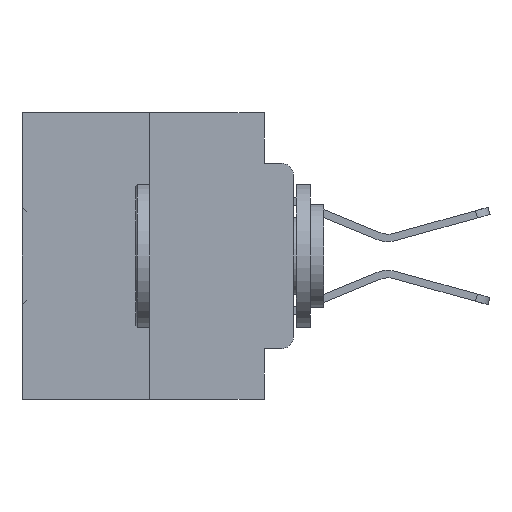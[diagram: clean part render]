
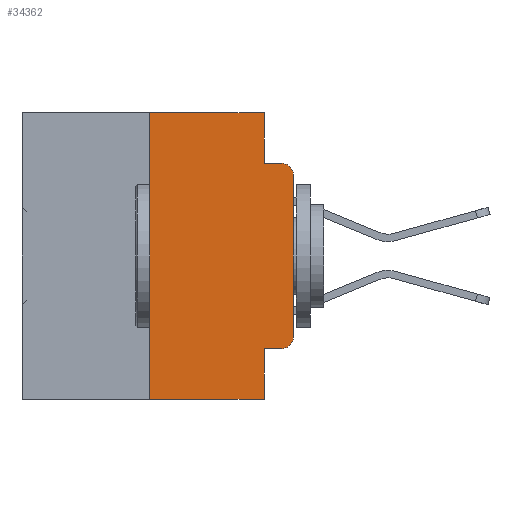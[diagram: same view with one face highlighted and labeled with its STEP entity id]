
A CAD part, left-side view. The second image highlights one B-rep face of the part: STEP entity #34362.
In plain terms, the highlighted planar face has unit normal (-1, 0, 0).
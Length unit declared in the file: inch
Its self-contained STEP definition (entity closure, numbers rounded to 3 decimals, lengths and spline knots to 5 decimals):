
#99 = DIRECTION ( 'NONE',  ( 0., 0., 1. ) ) ;
#336 = VECTOR ( 'NONE', #27512, 39.37008 ) ;
#488 = ORIENTED_EDGE ( 'NONE', *, *, #18316, .F. ) ;
#864 = CARTESIAN_POINT ( 'NONE',  ( 0., 0.25, 0. ) ) ;
#1005 = CIRCLE ( 'NONE', #3862, 0.02 ) ;
#1542 = CARTESIAN_POINT ( 'NONE',  ( 0., 0.051, -0.4115 ) ) ;
#1606 = LINE ( 'NONE', #27075, #15407 ) ;
#1761 = CARTESIAN_POINT ( 'NONE',  ( 0., 0.473, 0. ) ) ;
#2473 = CARTESIAN_POINT ( 'NONE',  ( 0., 0.051, -0.0885 ) ) ;
#3862 = AXIS2_PLACEMENT_3D ( 'NONE', #26338, #10183, #29022 ) ;
#4087 = CARTESIAN_POINT ( 'NONE',  ( 0., 0.051, -0.5 ) ) ;
#4309 = LINE ( 'NONE', #27183, #23450 ) ;
#4738 = EDGE_CURVE ( 'NONE', #10977, #25583, #14763, .T. ) ;
#4956 = VERTEX_POINT ( 'NONE', #8646 ) ;
#5624 = DIRECTION ( 'NONE',  ( 0., -1., 0. ) ) ;
#5842 = CARTESIAN_POINT ( 'NONE',  ( 0., 0.25, 0. ) ) ;
#5891 = CARTESIAN_POINT ( 'NONE',  ( 0., 0., -0.1085 ) ) ;
#7770 = EDGE_CURVE ( 'NONE', #33714, #25583, #26780, .T. ) ;
#7923 = FACE_OUTER_BOUND ( 'NONE', #13157, .T. ) ;
#8646 = CARTESIAN_POINT ( 'NONE',  ( 0., 0.051, 0. ) ) ;
#9098 = PLANE ( 'NONE',  #11448 ) ;
#9118 = EDGE_CURVE ( 'NONE', #9549, #9960, #34623, .T. ) ;
#9549 = VERTEX_POINT ( 'NONE', #18414 ) ;
#9716 = DIRECTION ( 'NONE',  ( 0., 0., -1. ) ) ;
#9960 = VERTEX_POINT ( 'NONE', #864 ) ;
#10183 = DIRECTION ( 'NONE',  ( -1., 0., 0. ) ) ;
#10211 = DIRECTION ( 'NONE',  ( -1., 0., 0. ) ) ;
#10331 = LINE ( 'NONE', #15131, #23854 ) ;
#10973 = VECTOR ( 'NONE', #23343, 39.37008 ) ;
#10977 = VERTEX_POINT ( 'NONE', #2473 ) ;
#11111 = VERTEX_POINT ( 'NONE', #30180 ) ;
#11183 = CARTESIAN_POINT ( 'NONE',  ( 0., 0.473, -0.5 ) ) ;
#11448 = AXIS2_PLACEMENT_3D ( 'NONE', #33256, #27983, #11882 ) ;
#11882 = DIRECTION ( 'NONE',  ( 0., 0., -1. ) ) ;
#13157 = EDGE_LOOP ( 'NONE', ( #28555, #32274, #33945, #488, #24757, #33546, #28111, #25209, #21452, #19400 ) ) ;
#13485 = EDGE_CURVE ( 'NONE', #27352, #11111, #32422, .T. ) ;
#13628 = LINE ( 'NONE', #1761, #34175 ) ;
#13690 = DIRECTION ( 'NONE',  ( 0., 0., -1. ) ) ;
#13884 = VECTOR ( 'NONE', #20913, 39.37008 ) ;
#14763 = LINE ( 'NONE', #31662, #13884 ) ;
#15034 = EDGE_CURVE ( 'NONE', #9549, #23127, #21850, .T. ) ;
#15131 = CARTESIAN_POINT ( 'NONE',  ( 0., 0.051, 0. ) ) ;
#15407 = VECTOR ( 'NONE', #13690, 39.37008 ) ;
#16814 = AXIS2_PLACEMENT_3D ( 'NONE', #26361, #10211, #29046 ) ;
#16963 = EDGE_CURVE ( 'NONE', #33119, #33714, #4309, .T. ) ;
#17180 = EDGE_CURVE ( 'NONE', #27352, #23127, #10331, .T. ) ;
#18316 = EDGE_CURVE ( 'NONE', #4956, #10977, #1606, .T. ) ;
#18414 = CARTESIAN_POINT ( 'NONE',  ( 0., 0.25, -0.5 ) ) ;
#19400 = ORIENTED_EDGE ( 'NONE', *, *, #34592, .T. ) ;
#20514 = EDGE_CURVE ( 'NONE', #9960, #4956, #13628, .T. ) ;
#20876 = DIRECTION ( 'NONE',  ( 0., -1., 0. ) ) ;
#20913 = DIRECTION ( 'NONE',  ( 0., -1., 0. ) ) ;
#21452 = ORIENTED_EDGE ( 'NONE', *, *, #13485, .T. ) ;
#21850 = LINE ( 'NONE', #11183, #28118 ) ;
#23127 = VERTEX_POINT ( 'NONE', #4087 ) ;
#23343 = DIRECTION ( 'NONE',  ( 0., -1., 0. ) ) ;
#23450 = VECTOR ( 'NONE', #99, 39.37008 ) ;
#23854 = VECTOR ( 'NONE', #9716, 39.37008 ) ;
#24539 = CARTESIAN_POINT ( 'NONE',  ( 0., 0.051, -0.4115 ) ) ;
#24757 = ORIENTED_EDGE ( 'NONE', *, *, #20514, .F. ) ;
#25146 = CARTESIAN_POINT ( 'NONE',  ( 0., 0., -0.3915 ) ) ;
#25209 = ORIENTED_EDGE ( 'NONE', *, *, #17180, .F. ) ;
#25583 = VERTEX_POINT ( 'NONE', #28491 ) ;
#26338 = CARTESIAN_POINT ( 'NONE',  ( 0., 0.02, -0.3915 ) ) ;
#26361 = CARTESIAN_POINT ( 'NONE',  ( 0., 0.02, -0.1085 ) ) ;
#26780 = CIRCLE ( 'NONE', #16814, 0.02 ) ;
#27075 = CARTESIAN_POINT ( 'NONE',  ( 0., 0.051, 0. ) ) ;
#27183 = CARTESIAN_POINT ( 'NONE',  ( 0., 0., 0. ) ) ;
#27352 = VERTEX_POINT ( 'NONE', #24539 ) ;
#27512 = DIRECTION ( 'NONE',  ( 0., 0., 1. ) ) ;
#27983 = DIRECTION ( 'NONE',  ( 1., 0., 0. ) ) ;
#28111 = ORIENTED_EDGE ( 'NONE', *, *, #15034, .T. ) ;
#28118 = VECTOR ( 'NONE', #5624, 39.37008 ) ;
#28491 = CARTESIAN_POINT ( 'NONE',  ( 0., 0.02, -0.0885 ) ) ;
#28555 = ORIENTED_EDGE ( 'NONE', *, *, #16963, .T. ) ;
#29022 = DIRECTION ( 'NONE',  ( 0., 0., -1. ) ) ;
#29046 = DIRECTION ( 'NONE',  ( 0., 0., -1. ) ) ;
#30180 = CARTESIAN_POINT ( 'NONE',  ( 0., 0.02, -0.4115 ) ) ;
#31662 = CARTESIAN_POINT ( 'NONE',  ( 0., 0.051, -0.0885 ) ) ;
#32274 = ORIENTED_EDGE ( 'NONE', *, *, #7770, .T. ) ;
#32422 = LINE ( 'NONE', #1542, #10973 ) ;
#33119 = VERTEX_POINT ( 'NONE', #25146 ) ;
#33256 = CARTESIAN_POINT ( 'NONE',  ( 0., 0.473, 0. ) ) ;
#33546 = ORIENTED_EDGE ( 'NONE', *, *, #9118, .F. ) ;
#33714 = VERTEX_POINT ( 'NONE', #5891 ) ;
#33945 = ORIENTED_EDGE ( 'NONE', *, *, #4738, .F. ) ;
#34175 = VECTOR ( 'NONE', #20876, 39.37008 ) ;
#34362 = ADVANCED_FACE ( 'NONE', ( #7923 ), #9098, .F. ) ;
#34592 = EDGE_CURVE ( 'NONE', #11111, #33119, #1005, .T. ) ;
#34623 = LINE ( 'NONE', #5842, #336 ) ;
